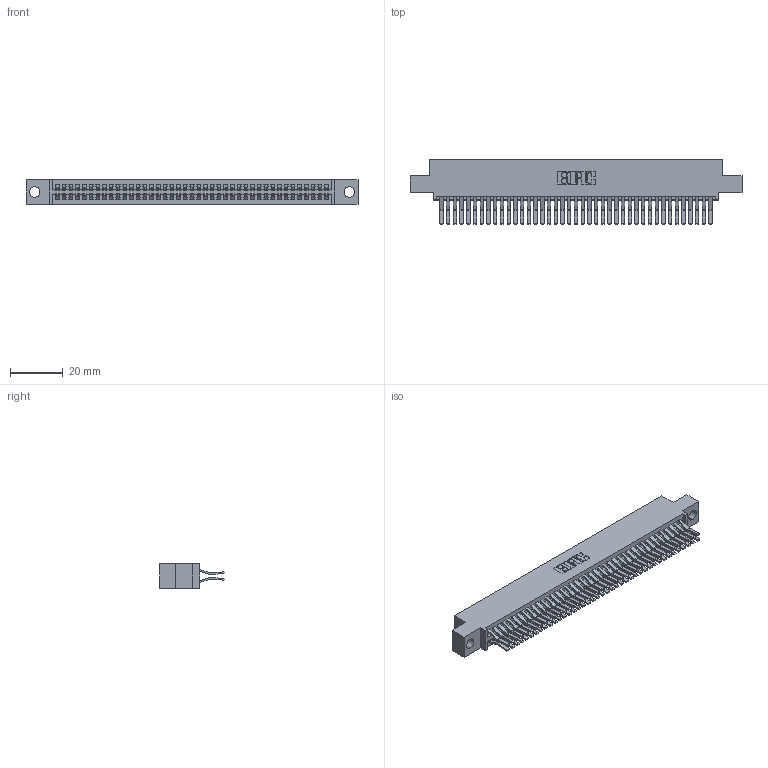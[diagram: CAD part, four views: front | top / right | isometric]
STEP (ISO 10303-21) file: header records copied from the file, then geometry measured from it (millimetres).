
FILE_DESCRIPTION (( 'STEP AP203' ), '1' );
FILE_NAME ('395-082-560-504.STEP', '2018-11-28T10:30:06', ( '' ), ( '' ), 'SwSTEP 2.0', 'SolidWorks 2016', '' );
FILE_SCHEMA (( 'CONFIG_CONTROL_DESIGN' ));
Length unit declared in the file: inch
Products named in the file (3): 395-082-560-504; 345-292-001_560 Tail; 345 Part_0.110 Offset - 0.156 Dia-TH
Assembly tree (83 placements, depth 2):
  395-082-560-504
    345 Part_0.110 Offset - 0.156 Dia-TH
    345-292-001_560 Tail  x82
Bounding box: 125.35 x 24.45 x 9.4 mm (x, y, z)
Volume: 12543.5 mm3; surface area: 19812.4 mm2
Topology: 83 solids, 83 shells, 4394 faces, 13063 edges, 8598 vertices
Faces by surface type: plane 2790, cylinder 1604
Entity records: 32527 total; most frequent: CARTESIAN_POINT 5456, ORIENTED_EDGE 5390, DIRECTION 4815, EDGE_CURVE 2695, VECTOR 2395, LINE 2395, VERTEX_POINT 1794, AXIS2_PLACEMENT_3D 1210
